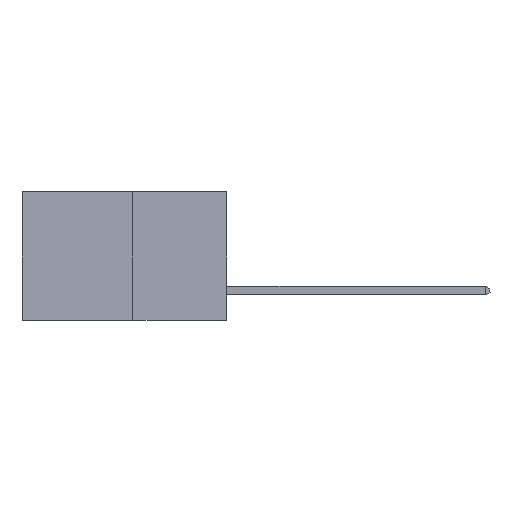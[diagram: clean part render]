
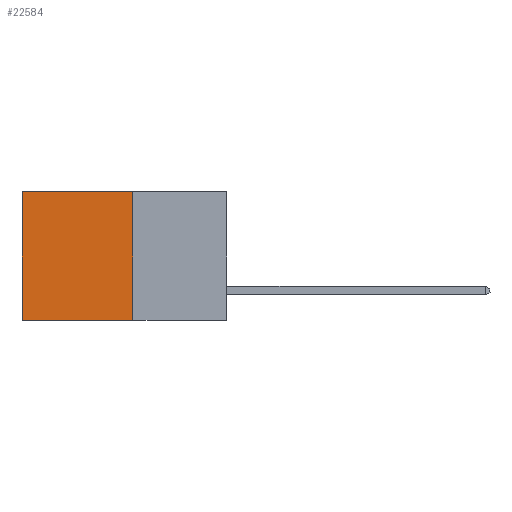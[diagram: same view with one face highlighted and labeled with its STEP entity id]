
A CAD part, left-side view. The second image highlights one B-rep face of the part: STEP entity #22584.
In plain terms, the highlighted planar face has unit normal (-1, 0, 0).
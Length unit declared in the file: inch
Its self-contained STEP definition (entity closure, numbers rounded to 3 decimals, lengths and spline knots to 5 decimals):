
#757 = DIRECTION ( 'NONE',  ( 0., 0., -1. ) ) ;
#1088 = LINE ( 'NONE', #5662, #5901 ) ;
#1671 = DIRECTION ( 'NONE',  ( 0., 1., 0. ) ) ;
#2083 = ORIENTED_EDGE ( 'NONE', *, *, #18329, .F. ) ;
#2363 = VERTEX_POINT ( 'NONE', #3276 ) ;
#2886 = VECTOR ( 'NONE', #17268, 39.37008 ) ;
#3276 = CARTESIAN_POINT ( 'NONE',  ( 0.277, 0.27, 0. ) ) ;
#3929 = CARTESIAN_POINT ( 'NONE',  ( 0.277, 0.27, -0.37 ) ) ;
#4337 = CARTESIAN_POINT ( 'NONE',  ( 0.277, 0.27, -0.37 ) ) ;
#5662 = CARTESIAN_POINT ( 'NONE',  ( 0.277, 0.59, -0.37 ) ) ;
#5741 = DIRECTION ( 'NONE',  ( 1., 0., 0. ) ) ;
#5901 = VECTOR ( 'NONE', #5966, 39.37008 ) ;
#5966 = DIRECTION ( 'NONE',  ( 0., 0., -1. ) ) ;
#6243 = EDGE_CURVE ( 'NONE', #13381, #17740, #1088, .T. ) ;
#7249 = VECTOR ( 'NONE', #1671, 39.37008 ) ;
#7710 = LINE ( 'NONE', #17193, #2886 ) ;
#7926 = EDGE_LOOP ( 'NONE', ( #9202, #8064, #2083, #15777 ) ) ;
#8064 = ORIENTED_EDGE ( 'NONE', *, *, #8442, .F. ) ;
#8442 = EDGE_CURVE ( 'NONE', #18827, #17740, #16104, .T. ) ;
#9202 = ORIENTED_EDGE ( 'NONE', *, *, #6243, .T. ) ;
#9892 = CARTESIAN_POINT ( 'NONE',  ( 0.277, 0.59, 0. ) ) ;
#12968 = AXIS2_PLACEMENT_3D ( 'NONE', #3929, #5741, #18104 ) ;
#13373 = FACE_OUTER_BOUND ( 'NONE', #7926, .T. ) ;
#13381 = VERTEX_POINT ( 'NONE', #9892 ) ;
#14596 = PLANE ( 'NONE',  #12968 ) ;
#15777 = ORIENTED_EDGE ( 'NONE', *, *, #17234, .T. ) ;
#16104 = LINE ( 'NONE', #22872, #7249 ) ;
#17193 = CARTESIAN_POINT ( 'NONE',  ( 0.277, 0.27, 0. ) ) ;
#17234 = EDGE_CURVE ( 'NONE', #2363, #13381, #7710, .T. ) ;
#17268 = DIRECTION ( 'NONE',  ( 0., 1., 0. ) ) ;
#17426 = VECTOR ( 'NONE', #757, 39.37008 ) ;
#17740 = VERTEX_POINT ( 'NONE', #18583 ) ;
#18104 = DIRECTION ( 'NONE',  ( 0., 0., -1. ) ) ;
#18329 = EDGE_CURVE ( 'NONE', #2363, #18827, #22040, .T. ) ;
#18583 = CARTESIAN_POINT ( 'NONE',  ( 0.277, 0.59, -0.37 ) ) ;
#18827 = VERTEX_POINT ( 'NONE', #22741 ) ;
#22040 = LINE ( 'NONE', #4337, #17426 ) ;
#22584 = ADVANCED_FACE ( 'NONE', ( #13373 ), #14596, .F. ) ;
#22741 = CARTESIAN_POINT ( 'NONE',  ( 0.277, 0.27, -0.37 ) ) ;
#22872 = CARTESIAN_POINT ( 'NONE',  ( 0.277, 0.27, -0.37 ) ) ;
